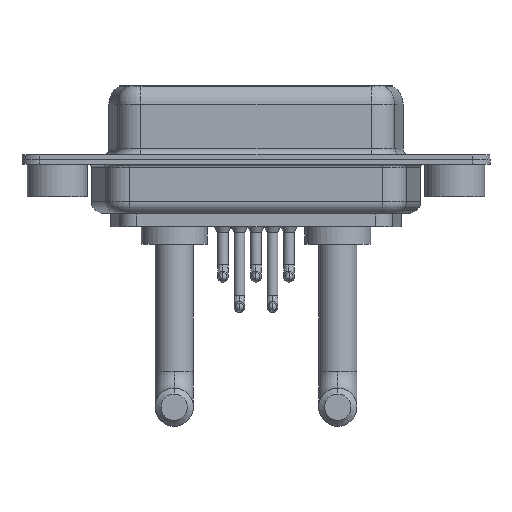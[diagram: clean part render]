
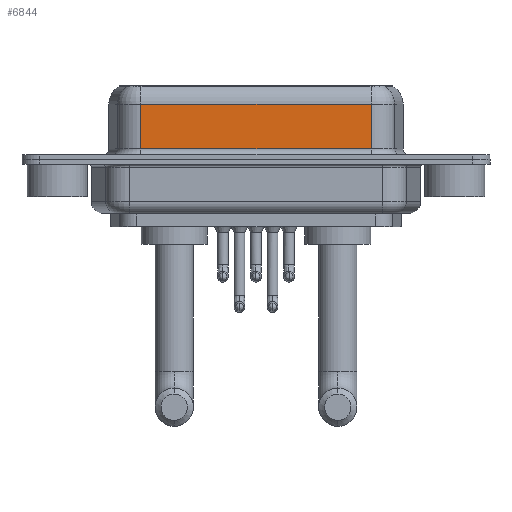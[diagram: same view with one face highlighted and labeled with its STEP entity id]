
A CAD part, front view. The second image highlights one B-rep face of the part: STEP entity #6844.
In plain terms, the highlighted planar face has unit normal (0, -1, 0).
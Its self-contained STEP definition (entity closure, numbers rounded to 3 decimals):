
#481 = VERTEX_POINT ( 'NONE', #4813 ) ;
#514 = CARTESIAN_POINT ( 'NONE',  ( 7.013, -3.95, 0.9 ) ) ;
#761 = DIRECTION ( 'NONE',  ( 0., 1., 0. ) ) ;
#866 = ORIENTED_EDGE ( 'NONE', *, *, #13314, .T. ) ;
#963 = AXIS2_PLACEMENT_3D ( 'NONE', #3080, #761, #16183 ) ;
#1707 = VECTOR ( 'NONE', #9704, 1000. ) ;
#1965 = LINE ( 'NONE', #4456, #14793 ) ;
#2436 = ORIENTED_EDGE ( 'NONE', *, *, #7256, .F. ) ;
#3080 = CARTESIAN_POINT ( 'NONE',  ( 26.287, -3.95, 6.4 ) ) ;
#3203 = CARTESIAN_POINT ( 'NONE',  ( 26.287, -3.95, 4.65 ) ) ;
#3378 = VERTEX_POINT ( 'NONE', #514 ) ;
#3689 = CARTESIAN_POINT ( 'NONE',  ( 7.013, -3.95, 6.4 ) ) ;
#3953 = CARTESIAN_POINT ( 'NONE',  ( 26.287, -3.95, 0.9 ) ) ;
#4456 = CARTESIAN_POINT ( 'NONE',  ( 26.287, -3.95, 6.4 ) ) ;
#4813 = CARTESIAN_POINT ( 'NONE',  ( 7.013, -3.95, 4.65 ) ) ;
#6844 = ADVANCED_FACE ( 'NONE', ( #12411 ), #8392, .F. ) ;
#7256 = EDGE_CURVE ( 'NONE', #8231, #9832, #1965, .T. ) ;
#7765 = CARTESIAN_POINT ( 'NONE',  ( 26.287, -3.95, 4.65 ) ) ;
#7798 = VECTOR ( 'NONE', #13203, 1000. ) ;
#8231 = VERTEX_POINT ( 'NONE', #7765 ) ;
#8392 = PLANE ( 'NONE',  #963 ) ;
#9419 = EDGE_LOOP ( 'NONE', ( #2436, #16507, #866, #11094 ) ) ;
#9553 = CARTESIAN_POINT ( 'NONE',  ( 26.287, -3.95, 0.9 ) ) ;
#9704 = DIRECTION ( 'NONE',  ( -1., 0., 0. ) ) ;
#9832 = VERTEX_POINT ( 'NONE', #9553 ) ;
#11094 = ORIENTED_EDGE ( 'NONE', *, *, #15219, .T. ) ;
#11159 = DIRECTION ( 'NONE',  ( 0., 0., -1. ) ) ;
#11536 = EDGE_CURVE ( 'NONE', #8231, #481, #12362, .T. ) ;
#12362 = LINE ( 'NONE', #3203, #1707 ) ;
#12411 = FACE_OUTER_BOUND ( 'NONE', #9419, .T. ) ;
#13203 = DIRECTION ( 'NONE',  ( 1., 0., 0. ) ) ;
#13314 = EDGE_CURVE ( 'NONE', #481, #3378, #16293, .T. ) ;
#13619 = DIRECTION ( 'NONE',  ( 0., 0., -1. ) ) ;
#14063 = VECTOR ( 'NONE', #11159, 1000. ) ;
#14793 = VECTOR ( 'NONE', #13619, 1000. ) ;
#15219 = EDGE_CURVE ( 'NONE', #3378, #9832, #15428, .T. ) ;
#15428 = LINE ( 'NONE', #3953, #7798 ) ;
#16183 = DIRECTION ( 'NONE',  ( 0., 0., 1. ) ) ;
#16293 = LINE ( 'NONE', #3689, #14063 ) ;
#16507 = ORIENTED_EDGE ( 'NONE', *, *, #11536, .T. ) ;
